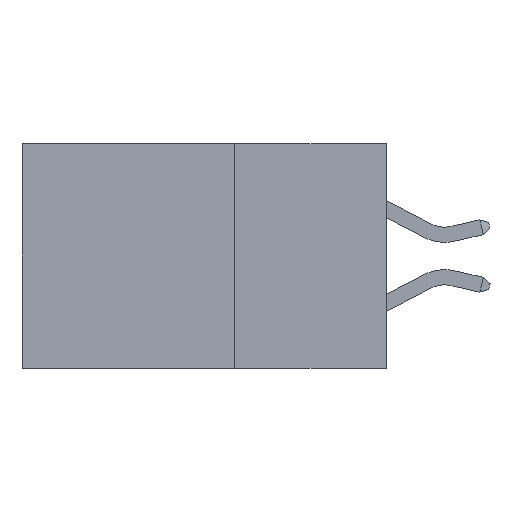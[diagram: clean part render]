
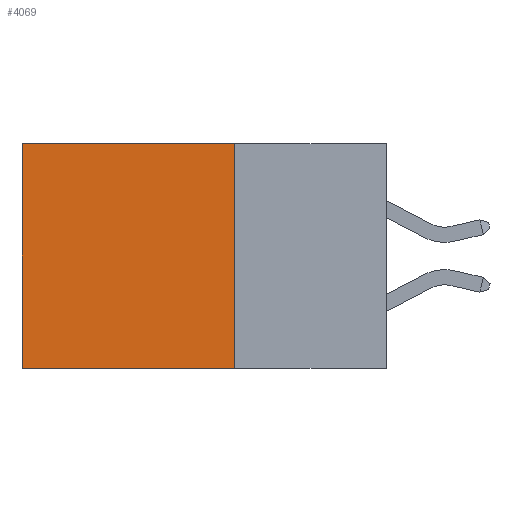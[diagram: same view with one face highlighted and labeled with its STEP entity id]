
A CAD part, left-side view. The second image highlights one B-rep face of the part: STEP entity #4069.
In plain terms, the highlighted planar face has unit normal (-1, 0, 0).
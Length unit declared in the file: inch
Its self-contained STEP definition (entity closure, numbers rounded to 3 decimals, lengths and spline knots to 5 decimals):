
#615 = CARTESIAN_POINT ( 'NONE',  ( 0.298, 0.25, -0.37 ) ) ;
#629 = ORIENTED_EDGE ( 'NONE', *, *, #19779, .F. ) ;
#1354 = EDGE_CURVE ( 'NONE', #15912, #11478, #11968, .T. ) ;
#1550 = DIRECTION ( 'NONE',  ( 0., 1., 0. ) ) ;
#1806 = CARTESIAN_POINT ( 'NONE',  ( 0.298, 0.6, -0.37 ) ) ;
#1852 = DIRECTION ( 'NONE',  ( 0., 0., -1. ) ) ;
#2436 = LINE ( 'NONE', #8550, #14473 ) ;
#2663 = LINE ( 'NONE', #9392, #9812 ) ;
#3274 = FACE_OUTER_BOUND ( 'NONE', #17956, .T. ) ;
#3349 = CARTESIAN_POINT ( 'NONE',  ( 0.298, 0.6, 0. ) ) ;
#3538 = VERTEX_POINT ( 'NONE', #615 ) ;
#3759 = LINE ( 'NONE', #5269, #9870 ) ;
#4023 = DIRECTION ( 'NONE',  ( 0., 0., -1. ) ) ;
#4069 = ADVANCED_FACE ( 'NONE', ( #3274 ), #10056, .F. ) ;
#5269 = CARTESIAN_POINT ( 'NONE',  ( 0.298, 0.25, 0. ) ) ;
#5480 = DIRECTION ( 'NONE',  ( 0., 0., -1. ) ) ;
#7733 = AXIS2_PLACEMENT_3D ( 'NONE', #18150, #16499, #4023 ) ;
#8108 = CARTESIAN_POINT ( 'NONE',  ( 0.298, 0.6, 0. ) ) ;
#8550 = CARTESIAN_POINT ( 'NONE',  ( 0.298, 0.25, 0. ) ) ;
#9392 = CARTESIAN_POINT ( 'NONE',  ( 0.298, 0.25, -0.37 ) ) ;
#9812 = VECTOR ( 'NONE', #1550, 39.37008 ) ;
#9870 = VECTOR ( 'NONE', #5480, 39.37008 ) ;
#10056 = PLANE ( 'NONE',  #7733 ) ;
#11376 = VERTEX_POINT ( 'NONE', #12157 ) ;
#11478 = VERTEX_POINT ( 'NONE', #1806 ) ;
#11968 = LINE ( 'NONE', #8108, #19870 ) ;
#12157 = CARTESIAN_POINT ( 'NONE',  ( 0.298, 0.25, 0. ) ) ;
#13261 = DIRECTION ( 'NONE',  ( 0., 1., 0. ) ) ;
#13941 = ORIENTED_EDGE ( 'NONE', *, *, #17660, .F. ) ;
#14473 = VECTOR ( 'NONE', #13261, 39.37008 ) ;
#15912 = VERTEX_POINT ( 'NONE', #3349 ) ;
#16499 = DIRECTION ( 'NONE',  ( 1., 0., 0. ) ) ;
#17660 = EDGE_CURVE ( 'NONE', #11376, #3538, #3759, .T. ) ;
#17956 = EDGE_LOOP ( 'NONE', ( #19577, #629, #13941, #18127 ) ) ;
#18127 = ORIENTED_EDGE ( 'NONE', *, *, #19096, .T. ) ;
#18150 = CARTESIAN_POINT ( 'NONE',  ( 0.298, 0.25, 0. ) ) ;
#19096 = EDGE_CURVE ( 'NONE', #11376, #15912, #2436, .T. ) ;
#19577 = ORIENTED_EDGE ( 'NONE', *, *, #1354, .T. ) ;
#19779 = EDGE_CURVE ( 'NONE', #3538, #11478, #2663, .T. ) ;
#19870 = VECTOR ( 'NONE', #1852, 39.37008 ) ;
